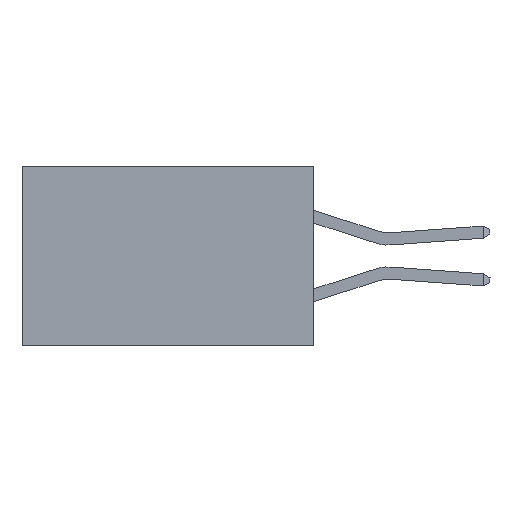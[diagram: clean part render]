
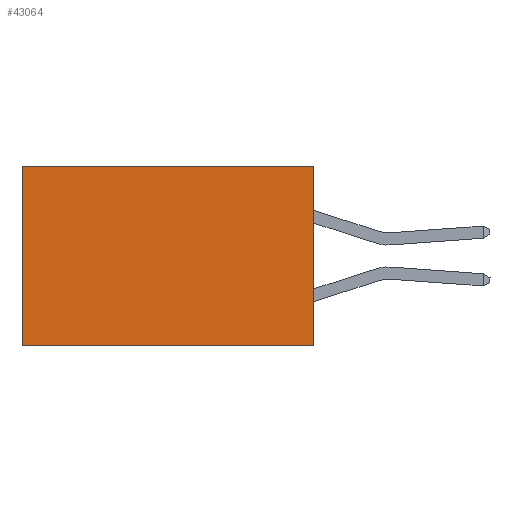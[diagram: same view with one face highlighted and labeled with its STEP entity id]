
A CAD part, left-side view. The second image highlights one B-rep face of the part: STEP entity #43064.
In plain terms, the highlighted planar face has unit normal (-1, 0, 0).
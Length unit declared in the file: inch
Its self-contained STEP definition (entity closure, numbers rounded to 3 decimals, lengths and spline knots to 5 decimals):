
#160 = DIRECTION ( 'NONE',  ( 0., 0., -1. ) ) ;
#1719 = VERTEX_POINT ( 'NONE', #42350 ) ;
#2896 = CARTESIAN_POINT ( 'NONE',  ( 0.2875, 0.6, 0. ) ) ;
#3647 = CARTESIAN_POINT ( 'NONE',  ( 0.2875, 0., 0. ) ) ;
#3921 = CARTESIAN_POINT ( 'NONE',  ( 0.2875, 0., -0.37 ) ) ;
#4737 = LINE ( 'NONE', #23258, #38092 ) ;
#4873 = ORIENTED_EDGE ( 'NONE', *, *, #12332, .F. ) ;
#6727 = DIRECTION ( 'NONE',  ( 1., 0., 0. ) ) ;
#10057 = EDGE_CURVE ( 'NONE', #13755, #1719, #43126, .T. ) ;
#11159 = DIRECTION ( 'NONE',  ( 0., 1., 0. ) ) ;
#11848 = EDGE_LOOP ( 'NONE', ( #40631, #12383, #4873, #28565 ) ) ;
#12332 = EDGE_CURVE ( 'NONE', #24941, #13755, #41344, .T. ) ;
#12383 = ORIENTED_EDGE ( 'NONE', *, *, #10057, .F. ) ;
#13373 = EDGE_CURVE ( 'NONE', #24941, #23741, #4737, .T. ) ;
#13444 = CARTESIAN_POINT ( 'NONE',  ( 0.2875, 0., 0. ) ) ;
#13755 = VERTEX_POINT ( 'NONE', #22504 ) ;
#21574 = CARTESIAN_POINT ( 'NONE',  ( 0.2875, 0.6, 0. ) ) ;
#21865 = AXIS2_PLACEMENT_3D ( 'NONE', #3647, #6727, #33631 ) ;
#22504 = CARTESIAN_POINT ( 'NONE',  ( 0.2875, 0., -0.37 ) ) ;
#23258 = CARTESIAN_POINT ( 'NONE',  ( 0.2875, 0., 0. ) ) ;
#23668 = DIRECTION ( 'NONE',  ( 0., 1., 0. ) ) ;
#23741 = VERTEX_POINT ( 'NONE', #21574 ) ;
#24941 = VERTEX_POINT ( 'NONE', #41537 ) ;
#26416 = VECTOR ( 'NONE', #11159, 39.37008 ) ;
#26750 = VECTOR ( 'NONE', #160, 39.37008 ) ;
#26935 = PLANE ( 'NONE',  #21865 ) ;
#28565 = ORIENTED_EDGE ( 'NONE', *, *, #13373, .T. ) ;
#32165 = FACE_OUTER_BOUND ( 'NONE', #11848, .T. ) ;
#32409 = VECTOR ( 'NONE', #42958, 39.37008 ) ;
#33631 = DIRECTION ( 'NONE',  ( 0., 0., -1. ) ) ;
#38092 = VECTOR ( 'NONE', #23668, 39.37008 ) ;
#39490 = EDGE_CURVE ( 'NONE', #23741, #1719, #41813, .T. ) ;
#40631 = ORIENTED_EDGE ( 'NONE', *, *, #39490, .T. ) ;
#41344 = LINE ( 'NONE', #13444, #26750 ) ;
#41537 = CARTESIAN_POINT ( 'NONE',  ( 0.2875, 0., 0. ) ) ;
#41813 = LINE ( 'NONE', #2896, #32409 ) ;
#42350 = CARTESIAN_POINT ( 'NONE',  ( 0.2875, 0.6, -0.37 ) ) ;
#42958 = DIRECTION ( 'NONE',  ( 0., 0., -1. ) ) ;
#43064 = ADVANCED_FACE ( 'NONE', ( #32165 ), #26935, .F. ) ;
#43126 = LINE ( 'NONE', #3921, #26416 ) ;
